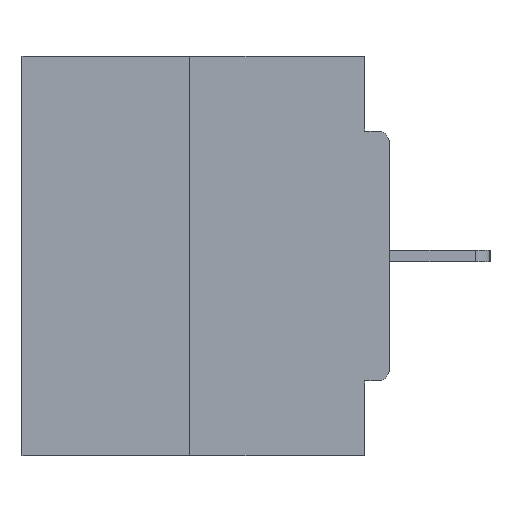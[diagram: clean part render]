
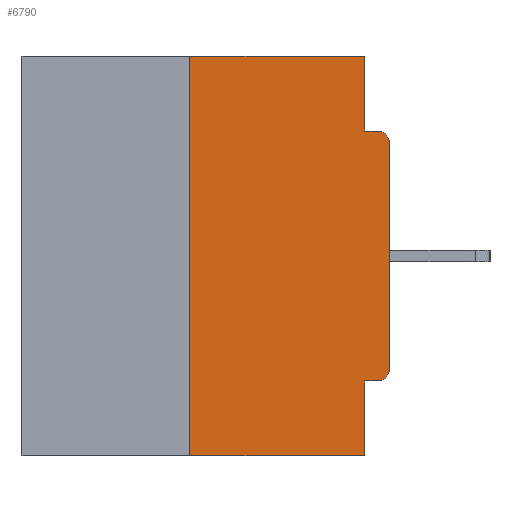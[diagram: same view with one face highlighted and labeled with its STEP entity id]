
A CAD part, left-side view. The second image highlights one B-rep face of the part: STEP entity #6790.
In plain terms, the highlighted planar face has unit normal (-1, 0, 0).
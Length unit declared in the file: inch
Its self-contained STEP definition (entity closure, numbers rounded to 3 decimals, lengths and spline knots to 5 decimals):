
#416 = VERTEX_POINT ( 'NONE', #2471 ) ;
#601 = VECTOR ( 'NONE', #17095, 39.37008 ) ;
#1006 = DIRECTION ( 'NONE',  ( 0., 0., -1. ) ) ;
#1052 = AXIS2_PLACEMENT_3D ( 'NONE', #23052, #21110, #1006 ) ;
#1211 = EDGE_CURVE ( 'NONE', #5602, #416, #14258, .T. ) ;
#1545 = EDGE_CURVE ( 'NONE', #10524, #26149, #10878, .T. ) ;
#1653 = DIRECTION ( 'NONE',  ( 0., -1., 0. ) ) ;
#1694 = DIRECTION ( 'NONE',  ( 0., 0., -1. ) ) ;
#1698 = ORIENTED_EDGE ( 'NONE', *, *, #17867, .T. ) ;
#1761 = LINE ( 'NONE', #6292, #7107 ) ;
#1767 = VERTEX_POINT ( 'NONE', #17694 ) ;
#2110 = DIRECTION ( 'NONE',  ( 0., -1., 0. ) ) ;
#2306 = VECTOR ( 'NONE', #2110, 39.37008 ) ;
#2471 = CARTESIAN_POINT ( 'NONE',  ( 0., 0.031, -0.0935 ) ) ;
#3070 = DIRECTION ( 'NONE',  ( 0., 0., -1. ) ) ;
#3787 = ORIENTED_EDGE ( 'NONE', *, *, #19020, .T. ) ;
#5391 = ORIENTED_EDGE ( 'NONE', *, *, #23102, .T. ) ;
#5602 = VERTEX_POINT ( 'NONE', #16866 ) ;
#5804 = EDGE_CURVE ( 'NONE', #16973, #5602, #1761, .T. ) ;
#6044 = CARTESIAN_POINT ( 'NONE',  ( 0., 0., -0.0935 ) ) ;
#6223 = ORIENTED_EDGE ( 'NONE', *, *, #23593, .F. ) ;
#6292 = CARTESIAN_POINT ( 'NONE',  ( 0., 0.46, 0. ) ) ;
#6790 = ADVANCED_FACE ( 'NONE', ( #24487 ), #22279, .F. ) ;
#7107 = VECTOR ( 'NONE', #15265, 39.37008 ) ;
#7109 = CARTESIAN_POINT ( 'NONE',  ( 0., 0.015, -0.0935 ) ) ;
#7465 = ORIENTED_EDGE ( 'NONE', *, *, #19270, .F. ) ;
#8190 = EDGE_CURVE ( 'NONE', #1767, #19319, #15420, .T. ) ;
#8348 = ORIENTED_EDGE ( 'NONE', *, *, #1545, .F. ) ;
#8357 = AXIS2_PLACEMENT_3D ( 'NONE', #8423, #10633, #1694 ) ;
#8423 = CARTESIAN_POINT ( 'NONE',  ( 0., 0.015, -0.3915 ) ) ;
#8757 = EDGE_CURVE ( 'NONE', #416, #25369, #12805, .T. ) ;
#9409 = CARTESIAN_POINT ( 'NONE',  ( 0., 0.031, -0.5 ) ) ;
#10029 = DIRECTION ( 'NONE',  ( 1., 0., 0. ) ) ;
#10524 = VERTEX_POINT ( 'NONE', #17195 ) ;
#10633 = DIRECTION ( 'NONE',  ( -1., 0., 0. ) ) ;
#10878 = LINE ( 'NONE', #13107, #11935 ) ;
#11479 = ORIENTED_EDGE ( 'NONE', *, *, #8190, .T. ) ;
#11935 = VECTOR ( 'NONE', #19832, 39.37008 ) ;
#12413 = VERTEX_POINT ( 'NONE', #25429 ) ;
#12805 = LINE ( 'NONE', #6044, #21450 ) ;
#13080 = LINE ( 'NONE', #13375, #23893 ) ;
#13107 = CARTESIAN_POINT ( 'NONE',  ( 0., 0.031, -0.5 ) ) ;
#13375 = CARTESIAN_POINT ( 'NONE',  ( 0., 0., 0. ) ) ;
#14258 = LINE ( 'NONE', #23208, #27452 ) ;
#14793 = AXIS2_PLACEMENT_3D ( 'NONE', #18690, #10029, #27994 ) ;
#15265 = DIRECTION ( 'NONE',  ( 0., -1., 0. ) ) ;
#15420 = CIRCLE ( 'NONE', #8357, 0.015 ) ;
#16866 = CARTESIAN_POINT ( 'NONE',  ( 0., 0.031, 0. ) ) ;
#16973 = VERTEX_POINT ( 'NONE', #23573 ) ;
#17095 = DIRECTION ( 'NONE',  ( 0., 1., 0. ) ) ;
#17148 = DIRECTION ( 'NONE',  ( 0., 0., 1. ) ) ;
#17195 = CARTESIAN_POINT ( 'NONE',  ( 0., 0.031, -0.4065 ) ) ;
#17465 = CIRCLE ( 'NONE', #1052, 0.015 ) ;
#17694 = CARTESIAN_POINT ( 'NONE',  ( 0., 0.015, -0.4065 ) ) ;
#17731 = CARTESIAN_POINT ( 'NONE',  ( 0., 0., -0.3915 ) ) ;
#17867 = EDGE_CURVE ( 'NONE', #19319, #28541, #13080, .T. ) ;
#18335 = EDGE_LOOP ( 'NONE', ( #22531, #7465, #3787, #8348, #6223, #11479, #1698, #5391, #20504, #21920 ) ) ;
#18690 = CARTESIAN_POINT ( 'NONE',  ( 0., 0.46, 0. ) ) ;
#19020 = EDGE_CURVE ( 'NONE', #12413, #26149, #21954, .T. ) ;
#19270 = EDGE_CURVE ( 'NONE', #12413, #16973, #28952, .T. ) ;
#19319 = VERTEX_POINT ( 'NONE', #17731 ) ;
#19626 = VECTOR ( 'NONE', #17148, 39.37008 ) ;
#19832 = DIRECTION ( 'NONE',  ( 0., 0., -1. ) ) ;
#20504 = ORIENTED_EDGE ( 'NONE', *, *, #8757, .F. ) ;
#21110 = DIRECTION ( 'NONE',  ( -1., 0., 0. ) ) ;
#21450 = VECTOR ( 'NONE', #1653, 39.37008 ) ;
#21920 = ORIENTED_EDGE ( 'NONE', *, *, #1211, .F. ) ;
#21954 = LINE ( 'NONE', #22240, #2306 ) ;
#22240 = CARTESIAN_POINT ( 'NONE',  ( 0., 0.46, -0.5 ) ) ;
#22279 = PLANE ( 'NONE',  #14793 ) ;
#22531 = ORIENTED_EDGE ( 'NONE', *, *, #5804, .F. ) ;
#23052 = CARTESIAN_POINT ( 'NONE',  ( 0., 0.015, -0.1085 ) ) ;
#23102 = EDGE_CURVE ( 'NONE', #28541, #25369, #17465, .T. ) ;
#23208 = CARTESIAN_POINT ( 'NONE',  ( 0., 0.031, 0. ) ) ;
#23573 = CARTESIAN_POINT ( 'NONE',  ( 0., 0.25, 0. ) ) ;
#23593 = EDGE_CURVE ( 'NONE', #1767, #10524, #28022, .T. ) ;
#23757 = CARTESIAN_POINT ( 'NONE',  ( 0., 0., -0.4065 ) ) ;
#23893 = VECTOR ( 'NONE', #29111, 39.37008 ) ;
#24099 = CARTESIAN_POINT ( 'NONE',  ( 0., 0.25, 0. ) ) ;
#24487 = FACE_OUTER_BOUND ( 'NONE', #18335, .T. ) ;
#25271 = CARTESIAN_POINT ( 'NONE',  ( 0., 0., -0.1085 ) ) ;
#25369 = VERTEX_POINT ( 'NONE', #7109 ) ;
#25429 = CARTESIAN_POINT ( 'NONE',  ( 0., 0.25, -0.5 ) ) ;
#26149 = VERTEX_POINT ( 'NONE', #9409 ) ;
#27452 = VECTOR ( 'NONE', #3070, 39.37008 ) ;
#27994 = DIRECTION ( 'NONE',  ( 0., 0., -1. ) ) ;
#28022 = LINE ( 'NONE', #23757, #601 ) ;
#28541 = VERTEX_POINT ( 'NONE', #25271 ) ;
#28952 = LINE ( 'NONE', #24099, #19626 ) ;
#29111 = DIRECTION ( 'NONE',  ( 0., 0., 1. ) ) ;
